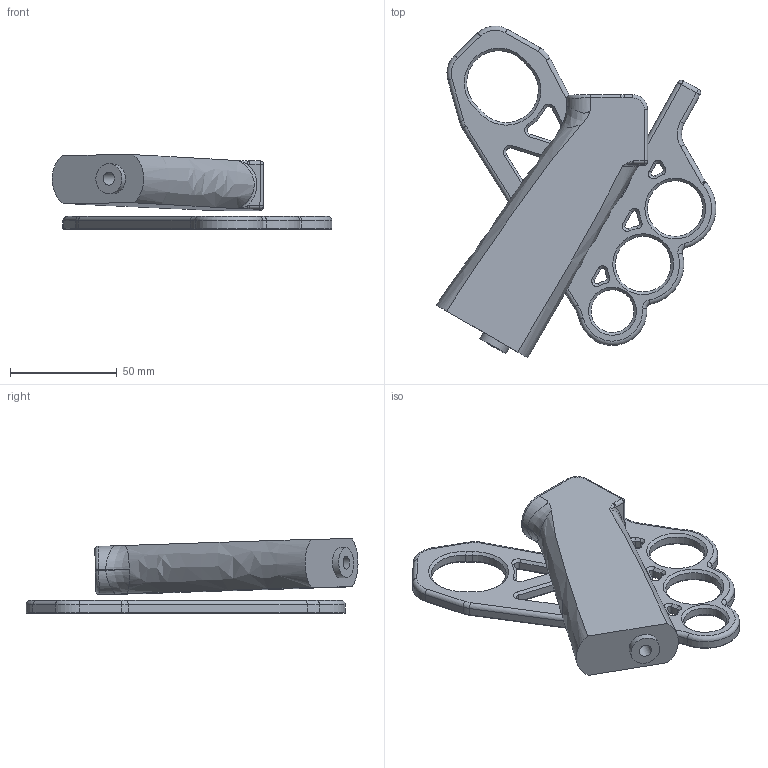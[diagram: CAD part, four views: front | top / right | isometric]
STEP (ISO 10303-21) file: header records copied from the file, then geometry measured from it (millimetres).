
FILE_DESCRIPTION(/* description */ (''),/* implementation_level */ '2;1');
FILE_NAME(/* name */ 'Gold Finger.stp',/* time_stamp */ '2022-01-18T09:36:16+02:00',/* author */ (''),/* organization */ (''),/* preprocessor_version */ 'ST-DEVELOPER v15.2',/* originating_system */ 'Autodesk Translator Framework v2.0.0.5431',/* authorisation */ '');
FILE_SCHEMA (('AUTOMOTIVE_DESIGN { 1 0 10303 214 3 1 1 }'));
Length unit declared in the file: centimetre
Products named in the file (1): (Unsaved)
Bounding box: 130.71 x 155.16 x 34.9 mm (x, y, z)
Volume: 141619.5 mm3; surface area: 37193.7 mm2
Topology: 2 solids, 2 shells, 267 faces, 631 edges, 367 vertices
Faces by surface type: cylinder 85, cone 65, plane 64, torus 34, bspline 15, sphere 4
Full cylindrical faces by diameter (mm): 3.8 x1, 6 x1, 14 x1, 20 x1, 26 x2
Entity records: 8885 total; most frequent: CARTESIAN_POINT 2693, DIRECTION 1381, ORIENTED_EDGE 1226, EDGE_CURVE 613, AXIS2_PLACEMENT_3D 546, VERTEX_POINT 364, EDGE_LOOP 303, LINE 289
